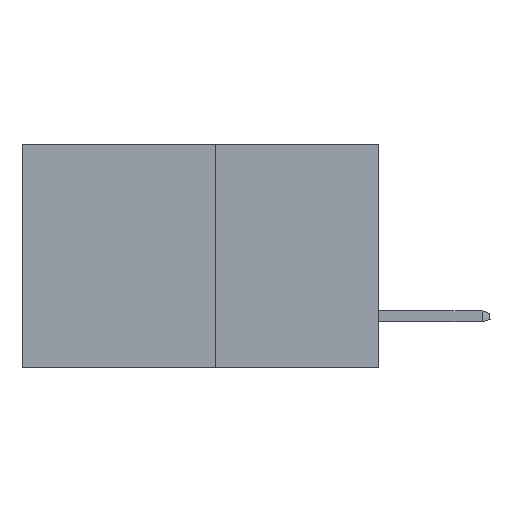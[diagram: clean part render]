
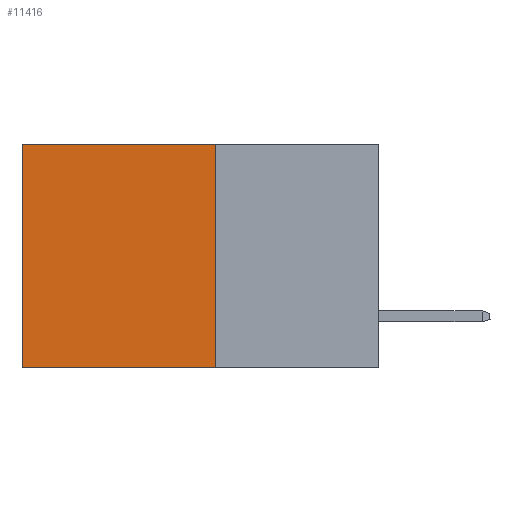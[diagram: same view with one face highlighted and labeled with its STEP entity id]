
A CAD part, left-side view. The second image highlights one B-rep face of the part: STEP entity #11416.
In plain terms, the highlighted planar face has unit normal (-1, 0, 0).
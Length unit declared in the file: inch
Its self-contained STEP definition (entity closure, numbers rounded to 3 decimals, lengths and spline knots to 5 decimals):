
#365 = CARTESIAN_POINT ( 'NONE',  ( 0.277, 0.27, -0.37 ) ) ;
#940 = CARTESIAN_POINT ( 'NONE',  ( 0.277, 0.59, -0.37 ) ) ;
#999 = ORIENTED_EDGE ( 'NONE', *, *, #16921, .T. ) ;
#1106 = DIRECTION ( 'NONE',  ( 0., 1., 0. ) ) ;
#1456 = VECTOR ( 'NONE', #12887, 39.37008 ) ;
#1679 = DIRECTION ( 'NONE',  ( 0., 1., 0. ) ) ;
#2183 = EDGE_LOOP ( 'NONE', ( #2836, #6752, #7197, #999 ) ) ;
#2836 = ORIENTED_EDGE ( 'NONE', *, *, #16704, .T. ) ;
#3650 = FACE_OUTER_BOUND ( 'NONE', #2183, .T. ) ;
#3775 = DIRECTION ( 'NONE',  ( 0., 0., -1. ) ) ;
#3812 = CARTESIAN_POINT ( 'NONE',  ( 0.277, 0.27, -0.37 ) ) ;
#4253 = VECTOR ( 'NONE', #1679, 39.37008 ) ;
#5555 = VECTOR ( 'NONE', #1106, 39.37008 ) ;
#5758 = VECTOR ( 'NONE', #16072, 39.37008 ) ;
#6672 = VERTEX_POINT ( 'NONE', #940 ) ;
#6752 = ORIENTED_EDGE ( 'NONE', *, *, #8882, .F. ) ;
#6952 = CARTESIAN_POINT ( 'NONE',  ( 0.277, 0.59, -0.37 ) ) ;
#7197 = ORIENTED_EDGE ( 'NONE', *, *, #15872, .F. ) ;
#7451 = CARTESIAN_POINT ( 'NONE',  ( 0.277, 0.59, 0. ) ) ;
#8837 = LINE ( 'NONE', #6952, #5758 ) ;
#8882 = EDGE_CURVE ( 'NONE', #15914, #6672, #14640, .T. ) ;
#8971 = CARTESIAN_POINT ( 'NONE',  ( 0.277, 0.27, -0.37 ) ) ;
#9021 = LINE ( 'NONE', #15455, #5555 ) ;
#10296 = VERTEX_POINT ( 'NONE', #10591 ) ;
#10591 = CARTESIAN_POINT ( 'NONE',  ( 0.277, 0.27, 0. ) ) ;
#11416 = ADVANCED_FACE ( 'NONE', ( #3650 ), #14142, .F. ) ;
#11601 = CARTESIAN_POINT ( 'NONE',  ( 0.277, 0.27, -0.37 ) ) ;
#11612 = DIRECTION ( 'NONE',  ( 1., 0., 0. ) ) ;
#11833 = VERTEX_POINT ( 'NONE', #7451 ) ;
#11925 = LINE ( 'NONE', #11601, #1456 ) ;
#12887 = DIRECTION ( 'NONE',  ( 0., 0., -1. ) ) ;
#14142 = PLANE ( 'NONE',  #14156 ) ;
#14156 = AXIS2_PLACEMENT_3D ( 'NONE', #8971, #11612, #3775 ) ;
#14640 = LINE ( 'NONE', #365, #4253 ) ;
#15455 = CARTESIAN_POINT ( 'NONE',  ( 0.277, 0.27, 0. ) ) ;
#15872 = EDGE_CURVE ( 'NONE', #10296, #15914, #11925, .T. ) ;
#15914 = VERTEX_POINT ( 'NONE', #3812 ) ;
#16072 = DIRECTION ( 'NONE',  ( 0., 0., -1. ) ) ;
#16704 = EDGE_CURVE ( 'NONE', #11833, #6672, #8837, .T. ) ;
#16921 = EDGE_CURVE ( 'NONE', #10296, #11833, #9021, .T. ) ;
